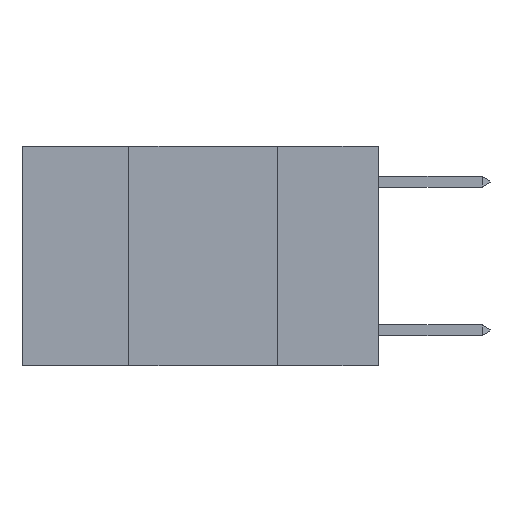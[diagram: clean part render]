
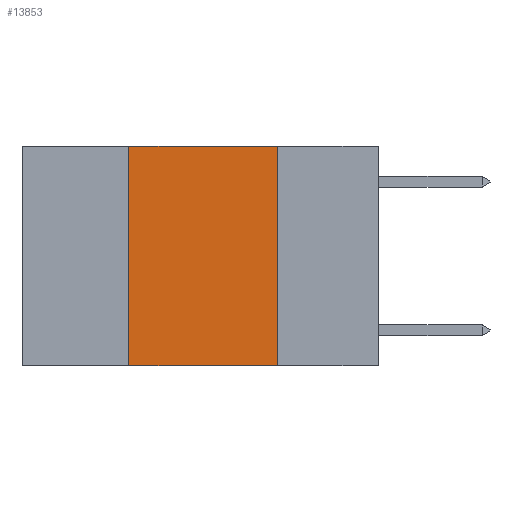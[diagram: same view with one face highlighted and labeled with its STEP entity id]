
A CAD part, left-side view. The second image highlights one B-rep face of the part: STEP entity #13853.
In plain terms, the highlighted planar face has unit normal (-1, 0, 0).
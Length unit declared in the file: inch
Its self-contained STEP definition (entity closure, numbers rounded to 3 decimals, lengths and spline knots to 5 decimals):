
#274 = VERTEX_POINT ( 'NONE', #22562 ) ;
#974 = VECTOR ( 'NONE', #11299, 39.37008 ) ;
#1278 = EDGE_CURVE ( 'NONE', #23381, #5829, #25052, .T. ) ;
#3138 = VECTOR ( 'NONE', #5309, 39.37008 ) ;
#5146 = EDGE_CURVE ( 'NONE', #5829, #274, #15252, .T. ) ;
#5309 = DIRECTION ( 'NONE',  ( 0., 0., 1. ) ) ;
#5324 = DIRECTION ( 'NONE',  ( 0., -1., 0. ) ) ;
#5829 = VERTEX_POINT ( 'NONE', #24262 ) ;
#6034 = LINE ( 'NONE', #24893, #24998 ) ;
#6331 = EDGE_CURVE ( 'NONE', #7079, #23381, #17070, .T. ) ;
#6536 = CARTESIAN_POINT ( 'NONE',  ( 0., 0.42, 0. ) ) ;
#7079 = VERTEX_POINT ( 'NONE', #19307 ) ;
#10337 = DIRECTION ( 'NONE',  ( 0., 0., -1. ) ) ;
#11299 = DIRECTION ( 'NONE',  ( 0., 0., -1. ) ) ;
#11955 = EDGE_LOOP ( 'NONE', ( #17577, #19296, #16527, #12264 ) ) ;
#12264 = ORIENTED_EDGE ( 'NONE', *, *, #21301, .T. ) ;
#13035 = CARTESIAN_POINT ( 'NONE',  ( 0., 0.6, 0. ) ) ;
#13158 = DIRECTION ( 'NONE',  ( 0., -1., 0. ) ) ;
#13853 = ADVANCED_FACE ( 'NONE', ( #17782 ), #15977, .F. ) ;
#15252 = LINE ( 'NONE', #24875, #974 ) ;
#15977 = PLANE ( 'NONE',  #21560 ) ;
#16527 = ORIENTED_EDGE ( 'NONE', *, *, #6331, .F. ) ;
#16959 = VECTOR ( 'NONE', #13158, 39.37008 ) ;
#17070 = LINE ( 'NONE', #24880, #3138 ) ;
#17577 = ORIENTED_EDGE ( 'NONE', *, *, #5146, .F. ) ;
#17782 = FACE_OUTER_BOUND ( 'NONE', #11955, .T. ) ;
#19296 = ORIENTED_EDGE ( 'NONE', *, *, #1278, .F. ) ;
#19307 = CARTESIAN_POINT ( 'NONE',  ( 0., 0.42, -0.37 ) ) ;
#21301 = EDGE_CURVE ( 'NONE', #7079, #274, #6034, .T. ) ;
#21560 = AXIS2_PLACEMENT_3D ( 'NONE', #23792, #21743, #10337 ) ;
#21743 = DIRECTION ( 'NONE',  ( 1., 0., 0. ) ) ;
#22562 = CARTESIAN_POINT ( 'NONE',  ( 0., 0.17, -0.37 ) ) ;
#23381 = VERTEX_POINT ( 'NONE', #6536 ) ;
#23792 = CARTESIAN_POINT ( 'NONE',  ( 0., 0.6, 0. ) ) ;
#24262 = CARTESIAN_POINT ( 'NONE',  ( 0., 0.17, 0. ) ) ;
#24875 = CARTESIAN_POINT ( 'NONE',  ( 0., 0.17, 0. ) ) ;
#24880 = CARTESIAN_POINT ( 'NONE',  ( 0., 0.42, 0. ) ) ;
#24893 = CARTESIAN_POINT ( 'NONE',  ( 0., 0.6, -0.37 ) ) ;
#24998 = VECTOR ( 'NONE', #5324, 39.37008 ) ;
#25052 = LINE ( 'NONE', #13035, #16959 ) ;
